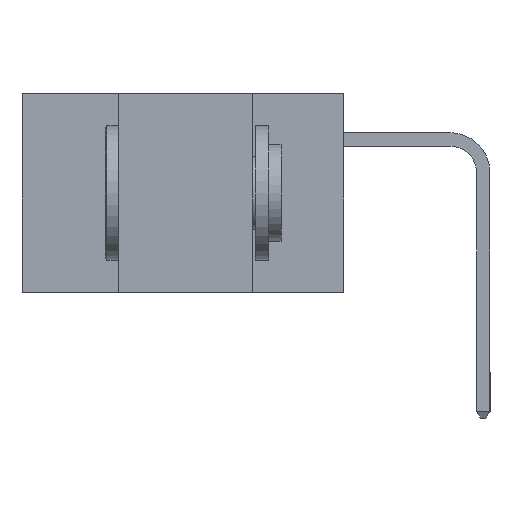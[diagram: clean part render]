
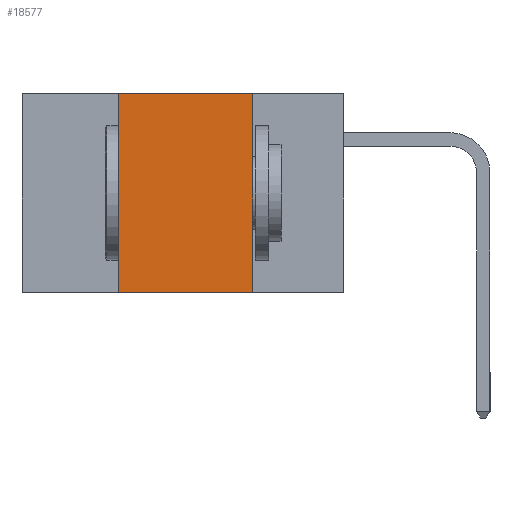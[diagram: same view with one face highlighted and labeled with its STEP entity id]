
A CAD part, left-side view. The second image highlights one B-rep face of the part: STEP entity #18577.
In plain terms, the highlighted planar face has unit normal (-1, 0, 0).
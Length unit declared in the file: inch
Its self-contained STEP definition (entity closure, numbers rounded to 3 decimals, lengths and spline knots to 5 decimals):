
#358 = DIRECTION ( 'NONE',  ( 0., -1., 0. ) ) ;
#379 = PLANE ( 'NONE',  #1704 ) ;
#1344 = VECTOR ( 'NONE', #2411, 39.37008 ) ;
#1704 = AXIS2_PLACEMENT_3D ( 'NONE', #15000, #8614, #12630 ) ;
#1929 = CARTESIAN_POINT ( 'NONE',  ( 0., 0.6, -0.37 ) ) ;
#2398 = EDGE_CURVE ( 'NONE', #15254, #18297, #4336, .T. ) ;
#2411 = DIRECTION ( 'NONE',  ( 0., 0., -1. ) ) ;
#3311 = VECTOR ( 'NONE', #4458, 39.37008 ) ;
#4095 = CARTESIAN_POINT ( 'NONE',  ( 0., 0.42, -0.37 ) ) ;
#4336 = LINE ( 'NONE', #1929, #5023 ) ;
#4458 = DIRECTION ( 'NONE',  ( 0., -1., 0. ) ) ;
#5023 = VECTOR ( 'NONE', #358, 39.37008 ) ;
#6477 = CARTESIAN_POINT ( 'NONE',  ( 0., 0.17, 0. ) ) ;
#7721 = FACE_OUTER_BOUND ( 'NONE', #18974, .T. ) ;
#8614 = DIRECTION ( 'NONE',  ( 1., 0., 0. ) ) ;
#11149 = LINE ( 'NONE', #6477, #1344 ) ;
#12630 = DIRECTION ( 'NONE',  ( 0., 0., -1. ) ) ;
#13088 = CARTESIAN_POINT ( 'NONE',  ( 0., 0.42, 0. ) ) ;
#13145 = LINE ( 'NONE', #19528, #21350 ) ;
#13728 = ORIENTED_EDGE ( 'NONE', *, *, #20891, .F. ) ;
#14009 = VERTEX_POINT ( 'NONE', #20241 ) ;
#14165 = ORIENTED_EDGE ( 'NONE', *, *, #26629, .F. ) ;
#14980 = EDGE_CURVE ( 'NONE', #15254, #25275, #13145, .T. ) ;
#15000 = CARTESIAN_POINT ( 'NONE',  ( 0., 0.6, 0. ) ) ;
#15168 = ORIENTED_EDGE ( 'NONE', *, *, #14980, .F. ) ;
#15254 = VERTEX_POINT ( 'NONE', #4095 ) ;
#16016 = ORIENTED_EDGE ( 'NONE', *, *, #2398, .T. ) ;
#17799 = CARTESIAN_POINT ( 'NONE',  ( 0., 0.17, -0.37 ) ) ;
#18297 = VERTEX_POINT ( 'NONE', #17799 ) ;
#18577 = ADVANCED_FACE ( 'NONE', ( #7721 ), #379, .F. ) ;
#18974 = EDGE_LOOP ( 'NONE', ( #14165, #13728, #15168, #16016 ) ) ;
#19011 = LINE ( 'NONE', #20909, #3311 ) ;
#19528 = CARTESIAN_POINT ( 'NONE',  ( 0., 0.42, 0. ) ) ;
#20241 = CARTESIAN_POINT ( 'NONE',  ( 0., 0.17, 0. ) ) ;
#20891 = EDGE_CURVE ( 'NONE', #25275, #14009, #19011, .T. ) ;
#20909 = CARTESIAN_POINT ( 'NONE',  ( 0., 0.6, 0. ) ) ;
#21350 = VECTOR ( 'NONE', #23858, 39.37008 ) ;
#23858 = DIRECTION ( 'NONE',  ( 0., 0., 1. ) ) ;
#25275 = VERTEX_POINT ( 'NONE', #13088 ) ;
#26629 = EDGE_CURVE ( 'NONE', #14009, #18297, #11149, .T. ) ;
